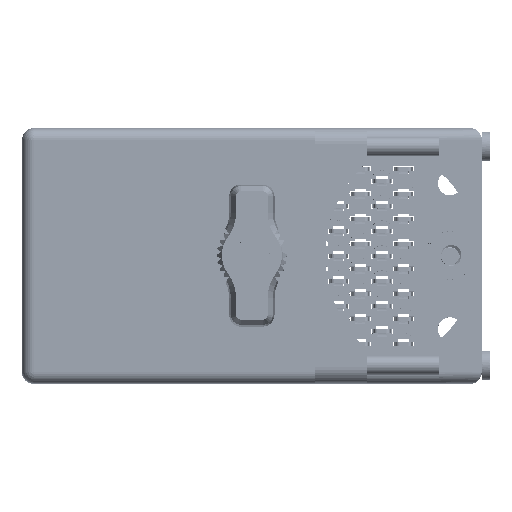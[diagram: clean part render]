
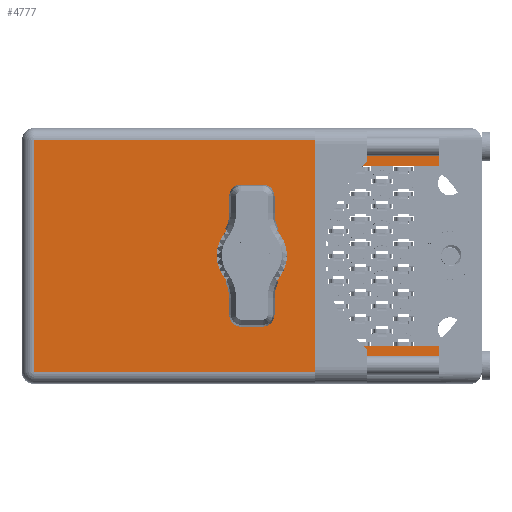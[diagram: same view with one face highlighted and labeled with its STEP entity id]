
A CAD part, top view. The second image highlights one B-rep face of the part: STEP entity #4777.
In plain terms, the highlighted face is planar.
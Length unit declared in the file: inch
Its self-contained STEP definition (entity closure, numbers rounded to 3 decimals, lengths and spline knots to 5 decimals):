
#852 = CARTESIAN_POINT ( 'NONE',  ( -1.3075, 1.93, -0.695 ) ) ;
#1035 = VERTEX_POINT ( 'NONE', #852 ) ;
#2410 = LINE ( 'NONE', #59019, #94778 ) ;
#3658 = CARTESIAN_POINT ( 'NONE',  ( 1.1215, 1.93, -0.765 ) ) ;
#3661 = CARTESIAN_POINT ( 'NONE',  ( 0., 1.93, -0.17 ) ) ;
#4672 = DIRECTION ( 'NONE',  ( 0., 0., 1. ) ) ;
#4777 = ADVANCED_FACE ( 'NONE', ( #60136, #11181 ), #54441, .T. ) ;
#8383 = VERTEX_POINT ( 'NONE', #105182 ) ;
#10965 = EDGE_CURVE ( 'NONE', #66586, #8383, #2410, .T. ) ;
#11181 = FACE_BOUND ( 'NONE', #43711, .T. ) ;
#12500 = DIRECTION ( 'NONE',  ( -1., 0., 0. ) ) ;
#12864 = VECTOR ( 'NONE', #12500, 39.37008 ) ;
#17070 = ORIENTED_EDGE ( 'NONE', *, *, #92033, .T. ) ;
#19891 = CARTESIAN_POINT ( 'NONE',  ( -1.3075, 1.93, -0.765 ) ) ;
#24349 = CIRCLE ( 'NONE', #62844, 0.17 ) ;
#24547 = EDGE_CURVE ( 'NONE', #62426, #68708, #92410, .T. ) ;
#26785 = CIRCLE ( 'NONE', #114961, 0.17 ) ;
#27263 = DIRECTION ( 'NONE',  ( 0., 0., 1. ) ) ;
#27975 = VERTEX_POINT ( 'NONE', #108635 ) ;
#28887 = DIRECTION ( 'NONE',  ( 0., 0., 1. ) ) ;
#29337 = DIRECTION ( 'NONE',  ( 0., 1., 0. ) ) ;
#30848 = ORIENTED_EDGE ( 'NONE', *, *, #66390, .T. ) ;
#30881 = EDGE_CURVE ( 'NONE', #47684, #8383, #62544, .T. ) ;
#32399 = DIRECTION ( 'NONE',  ( 0., 0., -1. ) ) ;
#32531 = ORIENTED_EDGE ( 'NONE', *, *, #76801, .F. ) ;
#34325 = ORIENTED_EDGE ( 'NONE', *, *, #50459, .F. ) ;
#35414 = VECTOR ( 'NONE', #28887, 39.37008 ) ;
#35555 = ORIENTED_EDGE ( 'NONE', *, *, #10965, .F. ) ;
#35980 = DIRECTION ( 'NONE',  ( 0., 0., 1. ) ) ;
#37725 = ORIENTED_EDGE ( 'NONE', *, *, #86565, .T. ) ;
#39501 = CARTESIAN_POINT ( 'NONE',  ( -1.3775, 1.93, -0.765 ) ) ;
#40356 = CARTESIAN_POINT ( 'NONE',  ( 0.4075, 1.93, -0.54 ) ) ;
#41422 = CARTESIAN_POINT ( 'NONE',  ( 1.1215, 1.93, 0.54 ) ) ;
#43711 = EDGE_LOOP ( 'NONE', ( #34325, #32531 ) ) ;
#47684 = VERTEX_POINT ( 'NONE', #40356 ) ;
#50459 = EDGE_CURVE ( 'NONE', #51912, #98672, #24349, .T. ) ;
#51912 = VERTEX_POINT ( 'NONE', #92461 ) ;
#53363 = DIRECTION ( 'NONE',  ( 1., 0., 0. ) ) ;
#54339 = EDGE_LOOP ( 'NONE', ( #37725, #30848, #55236, #85535, #17070, #90075, #35555, #79329 ) ) ;
#54441 = PLANE ( 'NONE',  #112573 ) ;
#54524 = CARTESIAN_POINT ( 'NONE',  ( 1.1215, 1.93, -0.54 ) ) ;
#54667 = CARTESIAN_POINT ( 'NONE',  ( 0., 1.93, 0. ) ) ;
#55236 = ORIENTED_EDGE ( 'NONE', *, *, #24547, .F. ) ;
#56037 = VECTOR ( 'NONE', #66752, 39.37008 ) ;
#56351 = DIRECTION ( 'NONE',  ( -1., 0., 0. ) ) ;
#57917 = DIRECTION ( 'NONE',  ( 1., 0., 0. ) ) ;
#58231 = VECTOR ( 'NONE', #53363, 39.37008 ) ;
#58962 = VECTOR ( 'NONE', #111226, 39.37008 ) ;
#59019 = CARTESIAN_POINT ( 'NONE',  ( 1.1215, 1.93, -0.765 ) ) ;
#59604 = CARTESIAN_POINT ( 'NONE',  ( 1.1215, 1.93, 0.695 ) ) ;
#60136 = FACE_OUTER_BOUND ( 'NONE', #54339, .T. ) ;
#62426 = VERTEX_POINT ( 'NONE', #41422 ) ;
#62544 = LINE ( 'NONE', #54524, #58231 ) ;
#62844 = AXIS2_PLACEMENT_3D ( 'NONE', #97334, #115346, #35980 ) ;
#66390 = EDGE_CURVE ( 'NONE', #27975, #68708, #74321, .T. ) ;
#66586 = VERTEX_POINT ( 'NONE', #85093 ) ;
#66752 = DIRECTION ( 'NONE',  ( -1., 0., 0. ) ) ;
#67215 = CARTESIAN_POINT ( 'NONE',  ( 0.4075, 1.93, -0.54 ) ) ;
#67701 = CARTESIAN_POINT ( 'NONE',  ( 1.1215, 1.93, 0.695 ) ) ;
#68708 = VERTEX_POINT ( 'NONE', #59604 ) ;
#70206 = EDGE_CURVE ( 'NONE', #62426, #76815, #92372, .T. ) ;
#73135 = LINE ( 'NONE', #19891, #35414 ) ;
#74321 = LINE ( 'NONE', #67701, #109370 ) ;
#76070 = CARTESIAN_POINT ( 'NONE',  ( 1.1215, 1.93, 0.54 ) ) ;
#76801 = EDGE_CURVE ( 'NONE', #98672, #51912, #26785, .T. ) ;
#76815 = VERTEX_POINT ( 'NONE', #80046 ) ;
#78297 = LINE ( 'NONE', #67215, #103568 ) ;
#79329 = ORIENTED_EDGE ( 'NONE', *, *, #89588, .T. ) ;
#80046 = CARTESIAN_POINT ( 'NONE',  ( 0.4075, 1.93, 0.54 ) ) ;
#80812 = DIRECTION ( 'NONE',  ( 0., 1., 0. ) ) ;
#85093 = CARTESIAN_POINT ( 'NONE',  ( 1.1215, 1.93, -0.695 ) ) ;
#85535 = ORIENTED_EDGE ( 'NONE', *, *, #70206, .T. ) ;
#86565 = EDGE_CURVE ( 'NONE', #1035, #27975, #73135, .T. ) ;
#89588 = EDGE_CURVE ( 'NONE', #66586, #1035, #105274, .T. ) ;
#90075 = ORIENTED_EDGE ( 'NONE', *, *, #30881, .T. ) ;
#92033 = EDGE_CURVE ( 'NONE', #76815, #47684, #78297, .T. ) ;
#92372 = LINE ( 'NONE', #76070, #56037 ) ;
#92410 = LINE ( 'NONE', #3658, #58962 ) ;
#92461 = CARTESIAN_POINT ( 'NONE',  ( 0., 1.93, 0.17 ) ) ;
#94778 = VECTOR ( 'NONE', #4672, 39.37008 ) ;
#97334 = CARTESIAN_POINT ( 'NONE',  ( 0., 1.93, 0. ) ) ;
#98672 = VERTEX_POINT ( 'NONE', #3661 ) ;
#103568 = VECTOR ( 'NONE', #32399, 39.37008 ) ;
#105182 = CARTESIAN_POINT ( 'NONE',  ( 1.1215, 1.93, -0.54 ) ) ;
#105274 = LINE ( 'NONE', #110298, #12864 ) ;
#108635 = CARTESIAN_POINT ( 'NONE',  ( -1.3075, 1.93, 0.695 ) ) ;
#109370 = VECTOR ( 'NONE', #57917, 39.37008 ) ;
#110298 = CARTESIAN_POINT ( 'NONE',  ( -1.3775, 1.93, -0.695 ) ) ;
#111226 = DIRECTION ( 'NONE',  ( 0., 0., 1. ) ) ;
#112573 = AXIS2_PLACEMENT_3D ( 'NONE', #39501, #29337, #56351 ) ;
#114961 = AXIS2_PLACEMENT_3D ( 'NONE', #54667, #80812, #27263 ) ;
#115346 = DIRECTION ( 'NONE',  ( 0., 1., 0. ) ) ;
